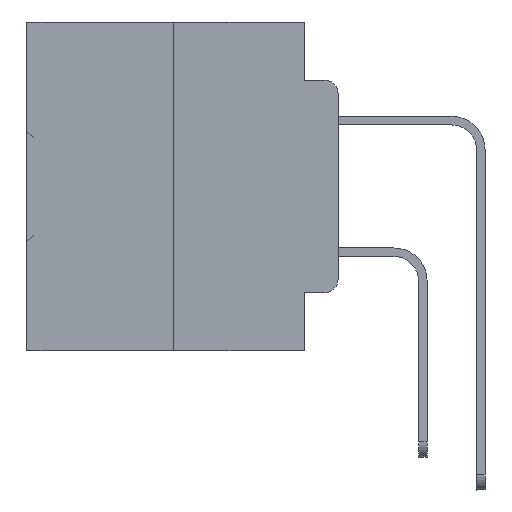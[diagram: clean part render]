
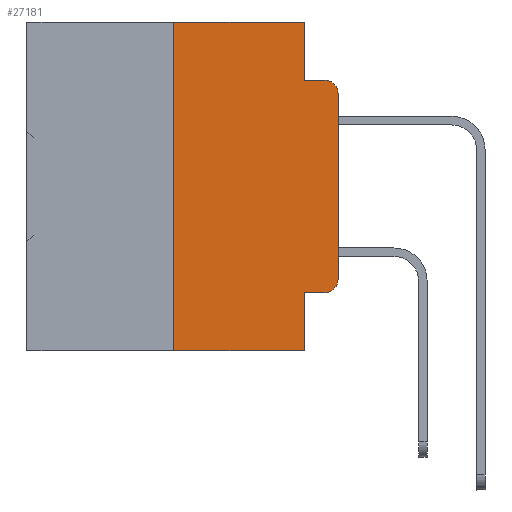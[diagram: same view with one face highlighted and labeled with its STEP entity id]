
A CAD part, left-side view. The second image highlights one B-rep face of the part: STEP entity #27181.
In plain terms, the highlighted planar face has unit normal (-1, 0, 0).
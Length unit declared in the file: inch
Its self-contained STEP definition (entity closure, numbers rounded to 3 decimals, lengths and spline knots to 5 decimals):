
#348 = CARTESIAN_POINT ( 'NONE',  ( 0., 0.051, 0. ) ) ;
#561 = ORIENTED_EDGE ( 'NONE', *, *, #15314, .T. ) ;
#2198 = CIRCLE ( 'NONE', #4782, 0.02 ) ;
#3094 = VERTEX_POINT ( 'NONE', #22214 ) ;
#3251 = CIRCLE ( 'NONE', #12200, 0.02 ) ;
#3695 = ORIENTED_EDGE ( 'NONE', *, *, #23543, .T. ) ;
#4782 = AXIS2_PLACEMENT_3D ( 'NONE', #27139, #29917, #33309 ) ;
#4852 = CARTESIAN_POINT ( 'NONE',  ( 0., 0.473, 0. ) ) ;
#5155 = EDGE_CURVE ( 'NONE', #25396, #30622, #37031, .T. ) ;
#5694 = CARTESIAN_POINT ( 'NONE',  ( 0., 0.051, -0.4115 ) ) ;
#6328 = DIRECTION ( 'NONE',  ( -1., 0., 0. ) ) ;
#7449 = LINE ( 'NONE', #16051, #20614 ) ;
#7890 = DIRECTION ( 'NONE',  ( 0., 0., -1. ) ) ;
#8184 = VERTEX_POINT ( 'NONE', #18580 ) ;
#8344 = VERTEX_POINT ( 'NONE', #348 ) ;
#8580 = ORIENTED_EDGE ( 'NONE', *, *, #9291, .F. ) ;
#9291 = EDGE_CURVE ( 'NONE', #8184, #14836, #25727, .T. ) ;
#9613 = EDGE_CURVE ( 'NONE', #3094, #35110, #22862, .T. ) ;
#9712 = VECTOR ( 'NONE', #16445, 39.37008 ) ;
#10410 = CARTESIAN_POINT ( 'NONE',  ( 0., 0.25, -0.5 ) ) ;
#10503 = DIRECTION ( 'NONE',  ( 0., 0., -1. ) ) ;
#12059 = ORIENTED_EDGE ( 'NONE', *, *, #13486, .F. ) ;
#12062 = VECTOR ( 'NONE', #35233, 39.37008 ) ;
#12200 = AXIS2_PLACEMENT_3D ( 'NONE', #15332, #6328, #33589 ) ;
#12508 = EDGE_LOOP ( 'NONE', ( #18721, #3695, #37216, #15468, #12059, #35650, #17544, #8580, #15234, #561 ) ) ;
#12800 = VERTEX_POINT ( 'NONE', #10410 ) ;
#12945 = EDGE_CURVE ( 'NONE', #12800, #14836, #17022, .T. ) ;
#13486 = EDGE_CURVE ( 'NONE', #28664, #8344, #18169, .T. ) ;
#13665 = FACE_OUTER_BOUND ( 'NONE', #12508, .T. ) ;
#14836 = VERTEX_POINT ( 'NONE', #33160 ) ;
#14998 = AXIS2_PLACEMENT_3D ( 'NONE', #4852, #38102, #22874 ) ;
#15021 = CARTESIAN_POINT ( 'NONE',  ( 0., 0.02, -0.0885 ) ) ;
#15234 = ORIENTED_EDGE ( 'NONE', *, *, #18492, .T. ) ;
#15314 = EDGE_CURVE ( 'NONE', #15840, #3094, #2198, .T. ) ;
#15332 = CARTESIAN_POINT ( 'NONE',  ( 0., 0.02, -0.1085 ) ) ;
#15468 = ORIENTED_EDGE ( 'NONE', *, *, #30011, .F. ) ;
#15840 = VERTEX_POINT ( 'NONE', #27659 ) ;
#16051 = CARTESIAN_POINT ( 'NONE',  ( 0., 0.25, 0. ) ) ;
#16445 = DIRECTION ( 'NONE',  ( 0., 0., 1. ) ) ;
#17022 = LINE ( 'NONE', #29629, #12062 ) ;
#17544 = ORIENTED_EDGE ( 'NONE', *, *, #12945, .T. ) ;
#18137 = DIRECTION ( 'NONE',  ( 0., -1., 0. ) ) ;
#18169 = LINE ( 'NONE', #35992, #20908 ) ;
#18492 = EDGE_CURVE ( 'NONE', #8184, #15840, #39538, .T. ) ;
#18580 = CARTESIAN_POINT ( 'NONE',  ( 0., 0.051, -0.4115 ) ) ;
#18721 = ORIENTED_EDGE ( 'NONE', *, *, #9613, .T. ) ;
#20614 = VECTOR ( 'NONE', #22679, 39.37008 ) ;
#20908 = VECTOR ( 'NONE', #35779, 39.37008 ) ;
#21204 = VECTOR ( 'NONE', #18137, 39.37008 ) ;
#21862 = VECTOR ( 'NONE', #10503, 39.37008 ) ;
#22214 = CARTESIAN_POINT ( 'NONE',  ( 0., 0., -0.3915 ) ) ;
#22679 = DIRECTION ( 'NONE',  ( 0., 0., 1. ) ) ;
#22862 = LINE ( 'NONE', #34289, #9712 ) ;
#22874 = DIRECTION ( 'NONE',  ( 0., 0., -1. ) ) ;
#22974 = VECTOR ( 'NONE', #34035, 39.37008 ) ;
#23096 = LINE ( 'NONE', #35318, #26228 ) ;
#23543 = EDGE_CURVE ( 'NONE', #35110, #30622, #3251, .T. ) ;
#25396 = VERTEX_POINT ( 'NONE', #25732 ) ;
#25727 = LINE ( 'NONE', #37952, #21862 ) ;
#25732 = CARTESIAN_POINT ( 'NONE',  ( 0., 0.051, -0.0885 ) ) ;
#26228 = VECTOR ( 'NONE', #7890, 39.37008 ) ;
#27139 = CARTESIAN_POINT ( 'NONE',  ( 0., 0.02, -0.3915 ) ) ;
#27178 = CARTESIAN_POINT ( 'NONE',  ( 0., 0., -0.1085 ) ) ;
#27181 = ADVANCED_FACE ( 'NONE', ( #13665 ), #32293, .F. ) ;
#27659 = CARTESIAN_POINT ( 'NONE',  ( 0., 0.02, -0.4115 ) ) ;
#28664 = VERTEX_POINT ( 'NONE', #34060 ) ;
#29629 = CARTESIAN_POINT ( 'NONE',  ( 0., 0.473, -0.5 ) ) ;
#29917 = DIRECTION ( 'NONE',  ( -1., 0., 0. ) ) ;
#30011 = EDGE_CURVE ( 'NONE', #8344, #25396, #23096, .T. ) ;
#30622 = VERTEX_POINT ( 'NONE', #15021 ) ;
#32293 = PLANE ( 'NONE',  #14998 ) ;
#33160 = CARTESIAN_POINT ( 'NONE',  ( 0., 0.051, -0.5 ) ) ;
#33309 = DIRECTION ( 'NONE',  ( 0., 0., -1. ) ) ;
#33589 = DIRECTION ( 'NONE',  ( 0., 0., -1. ) ) ;
#33659 = EDGE_CURVE ( 'NONE', #12800, #28664, #7449, .T. ) ;
#34035 = DIRECTION ( 'NONE',  ( 0., -1., 0. ) ) ;
#34060 = CARTESIAN_POINT ( 'NONE',  ( 0., 0.25, 0. ) ) ;
#34289 = CARTESIAN_POINT ( 'NONE',  ( 0., 0., 0. ) ) ;
#35110 = VERTEX_POINT ( 'NONE', #27178 ) ;
#35233 = DIRECTION ( 'NONE',  ( 0., -1., 0. ) ) ;
#35318 = CARTESIAN_POINT ( 'NONE',  ( 0., 0.051, 0. ) ) ;
#35650 = ORIENTED_EDGE ( 'NONE', *, *, #33659, .F. ) ;
#35779 = DIRECTION ( 'NONE',  ( 0., -1., 0. ) ) ;
#35992 = CARTESIAN_POINT ( 'NONE',  ( 0., 0.473, 0. ) ) ;
#36846 = CARTESIAN_POINT ( 'NONE',  ( 0., 0.051, -0.0885 ) ) ;
#37031 = LINE ( 'NONE', #36846, #22974 ) ;
#37216 = ORIENTED_EDGE ( 'NONE', *, *, #5155, .F. ) ;
#37952 = CARTESIAN_POINT ( 'NONE',  ( 0., 0.051, 0. ) ) ;
#38102 = DIRECTION ( 'NONE',  ( 1., 0., 0. ) ) ;
#39538 = LINE ( 'NONE', #5694, #21204 ) ;
